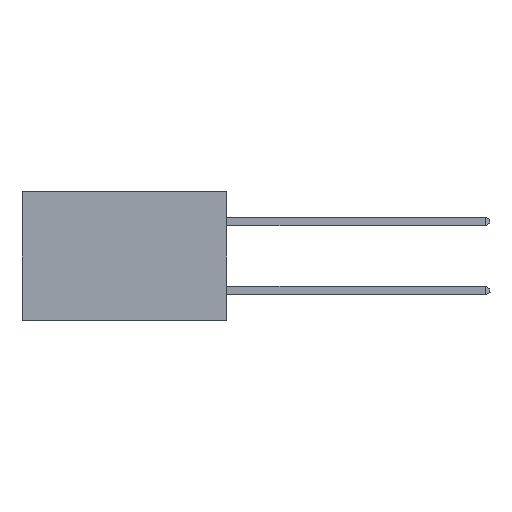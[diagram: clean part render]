
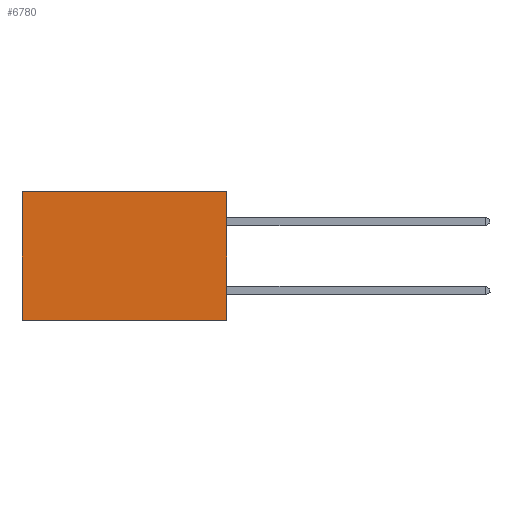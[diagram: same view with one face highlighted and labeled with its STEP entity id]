
A CAD part, left-side view. The second image highlights one B-rep face of the part: STEP entity #6780.
In plain terms, the highlighted planar face has unit normal (-1, 0, 0).
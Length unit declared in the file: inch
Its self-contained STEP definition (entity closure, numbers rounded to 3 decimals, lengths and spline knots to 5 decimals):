
#48 = ORIENTED_EDGE ( 'NONE', *, *, #8755, .T. ) ;
#1343 = VECTOR ( 'NONE', #7385, 39.37008 ) ;
#1493 = CARTESIAN_POINT ( 'NONE',  ( 0.277, 0.59, -0.37 ) ) ;
#1642 = LINE ( 'NONE', #12222, #10226 ) ;
#1736 = VERTEX_POINT ( 'NONE', #4352 ) ;
#1897 = ORIENTED_EDGE ( 'NONE', *, *, #10769, .F. ) ;
#2979 = ORIENTED_EDGE ( 'NONE', *, *, #8940, .T. ) ;
#3839 = VERTEX_POINT ( 'NONE', #8804 ) ;
#4072 = VERTEX_POINT ( 'NONE', #5275 ) ;
#4144 = DIRECTION ( 'NONE',  ( 0., 1., 0. ) ) ;
#4352 = CARTESIAN_POINT ( 'NONE',  ( 0.277, 0.59, 0. ) ) ;
#4466 = LINE ( 'NONE', #5025, #1343 ) ;
#5025 = CARTESIAN_POINT ( 'NONE',  ( 0.277, 0.59, -0.37 ) ) ;
#5088 = EDGE_CURVE ( 'NONE', #3839, #7503, #14657, .T. ) ;
#5275 = CARTESIAN_POINT ( 'NONE',  ( 0.277, 0., 0. ) ) ;
#6172 = AXIS2_PLACEMENT_3D ( 'NONE', #13507, #13366, #13354 ) ;
#6605 = EDGE_LOOP ( 'NONE', ( #48, #10459, #1897, #2979 ) ) ;
#6780 = ADVANCED_FACE ( 'NONE', ( #12996 ), #13489, .F. ) ;
#7385 = DIRECTION ( 'NONE',  ( 0., 0., -1. ) ) ;
#7503 = VERTEX_POINT ( 'NONE', #1493 ) ;
#8433 = VECTOR ( 'NONE', #9101, 39.37008 ) ;
#8487 = LINE ( 'NONE', #13581, #14355 ) ;
#8755 = EDGE_CURVE ( 'NONE', #1736, #7503, #4466, .T. ) ;
#8804 = CARTESIAN_POINT ( 'NONE',  ( 0.277, 0., -0.37 ) ) ;
#8940 = EDGE_CURVE ( 'NONE', #4072, #1736, #8487, .T. ) ;
#9087 = CARTESIAN_POINT ( 'NONE',  ( 0.277, 0., -0.37 ) ) ;
#9101 = DIRECTION ( 'NONE',  ( 0., 1., 0. ) ) ;
#10226 = VECTOR ( 'NONE', #13419, 39.37008 ) ;
#10459 = ORIENTED_EDGE ( 'NONE', *, *, #5088, .F. ) ;
#10769 = EDGE_CURVE ( 'NONE', #4072, #3839, #1642, .T. ) ;
#12222 = CARTESIAN_POINT ( 'NONE',  ( 0.277, 0., -0.37 ) ) ;
#12996 = FACE_OUTER_BOUND ( 'NONE', #6605, .T. ) ;
#13354 = DIRECTION ( 'NONE',  ( 0., 0., -1. ) ) ;
#13366 = DIRECTION ( 'NONE',  ( 1., 0., 0. ) ) ;
#13419 = DIRECTION ( 'NONE',  ( 0., 0., -1. ) ) ;
#13489 = PLANE ( 'NONE',  #6172 ) ;
#13507 = CARTESIAN_POINT ( 'NONE',  ( 0.277, 0., -0.37 ) ) ;
#13581 = CARTESIAN_POINT ( 'NONE',  ( 0.277, 0., 0. ) ) ;
#14355 = VECTOR ( 'NONE', #4144, 39.37008 ) ;
#14657 = LINE ( 'NONE', #9087, #8433 ) ;
